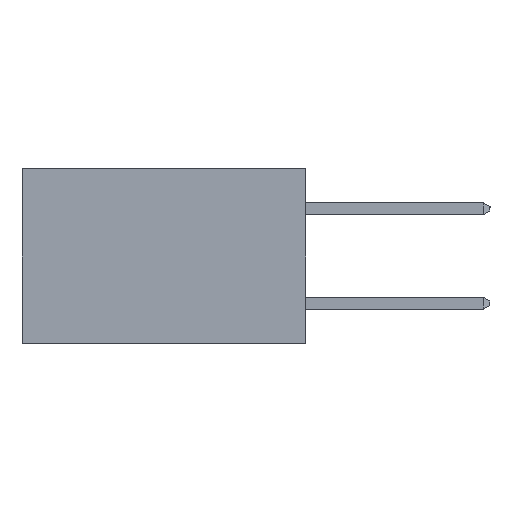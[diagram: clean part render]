
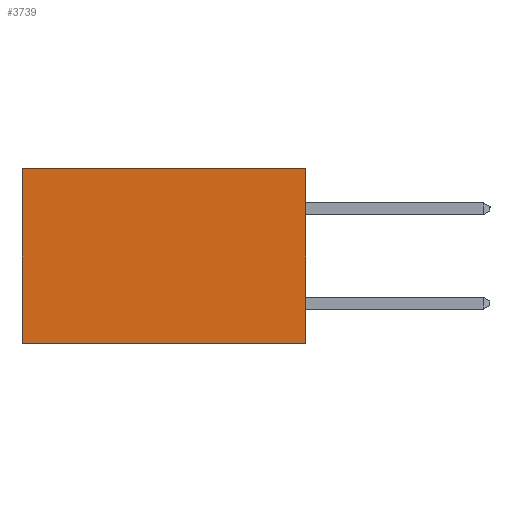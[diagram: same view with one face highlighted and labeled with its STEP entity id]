
A CAD part, left-side view. The second image highlights one B-rep face of the part: STEP entity #3739.
In plain terms, the highlighted planar face has unit normal (-1, 0, 0).
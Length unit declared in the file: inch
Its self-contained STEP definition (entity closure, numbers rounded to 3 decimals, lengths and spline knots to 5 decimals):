
#178 = VECTOR ( 'NONE', #5594, 39.37008 ) ;
#993 = CARTESIAN_POINT ( 'NONE',  ( 0.2615, 0., -0.37 ) ) ;
#1780 = DIRECTION ( 'NONE',  ( 1., 0., 0. ) ) ;
#2032 = LINE ( 'NONE', #16030, #178 ) ;
#2597 = LINE ( 'NONE', #993, #5223 ) ;
#2708 = DIRECTION ( 'NONE',  ( 0., 1., 0. ) ) ;
#3739 = ADVANCED_FACE ( 'NONE', ( #7052 ), #20829, .F. ) ;
#5097 = VERTEX_POINT ( 'NONE', #21321 ) ;
#5125 = ORIENTED_EDGE ( 'NONE', *, *, #15995, .F. ) ;
#5158 = EDGE_CURVE ( 'NONE', #5097, #16166, #2032, .T. ) ;
#5223 = VECTOR ( 'NONE', #2708, 39.37008 ) ;
#5594 = DIRECTION ( 'NONE',  ( 0., 1., 0. ) ) ;
#7052 = FACE_OUTER_BOUND ( 'NONE', #16077, .T. ) ;
#7169 = VERTEX_POINT ( 'NONE', #22006 ) ;
#8088 = VECTOR ( 'NONE', #9812, 39.37008 ) ;
#8429 = DIRECTION ( 'NONE',  ( 0., 0., -1. ) ) ;
#8887 = LINE ( 'NONE', #21301, #21606 ) ;
#9101 = ORIENTED_EDGE ( 'NONE', *, *, #5158, .T. ) ;
#9699 = CARTESIAN_POINT ( 'NONE',  ( 0.2615, 0., -0.37 ) ) ;
#9780 = CARTESIAN_POINT ( 'NONE',  ( 0.2615, 0., -0.37 ) ) ;
#9812 = DIRECTION ( 'NONE',  ( 0., 0., -1. ) ) ;
#12313 = VERTEX_POINT ( 'NONE', #9780 ) ;
#13983 = EDGE_CURVE ( 'NONE', #16166, #7169, #8887, .T. ) ;
#15640 = AXIS2_PLACEMENT_3D ( 'NONE', #17498, #1780, #8429 ) ;
#15995 = EDGE_CURVE ( 'NONE', #5097, #12313, #20387, .T. ) ;
#16030 = CARTESIAN_POINT ( 'NONE',  ( 0.2615, 0., 0. ) ) ;
#16077 = EDGE_LOOP ( 'NONE', ( #22463, #19509, #5125, #9101 ) ) ;
#16166 = VERTEX_POINT ( 'NONE', #20731 ) ;
#17498 = CARTESIAN_POINT ( 'NONE',  ( 0.2615, 0., -0.37 ) ) ;
#19509 = ORIENTED_EDGE ( 'NONE', *, *, #19752, .F. ) ;
#19695 = DIRECTION ( 'NONE',  ( 0., 0., -1. ) ) ;
#19752 = EDGE_CURVE ( 'NONE', #12313, #7169, #2597, .T. ) ;
#20387 = LINE ( 'NONE', #9699, #8088 ) ;
#20731 = CARTESIAN_POINT ( 'NONE',  ( 0.2615, 0.6, 0. ) ) ;
#20829 = PLANE ( 'NONE',  #15640 ) ;
#21301 = CARTESIAN_POINT ( 'NONE',  ( 0.2615, 0.6, -0.37 ) ) ;
#21321 = CARTESIAN_POINT ( 'NONE',  ( 0.2615, 0., 0. ) ) ;
#21606 = VECTOR ( 'NONE', #19695, 39.37008 ) ;
#22006 = CARTESIAN_POINT ( 'NONE',  ( 0.2615, 0.6, -0.37 ) ) ;
#22463 = ORIENTED_EDGE ( 'NONE', *, *, #13983, .T. ) ;
